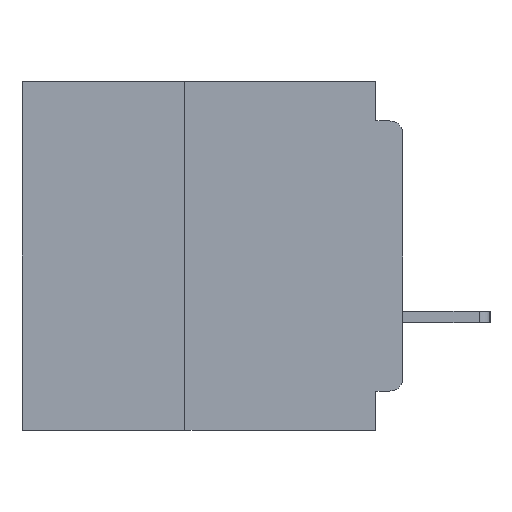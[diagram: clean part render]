
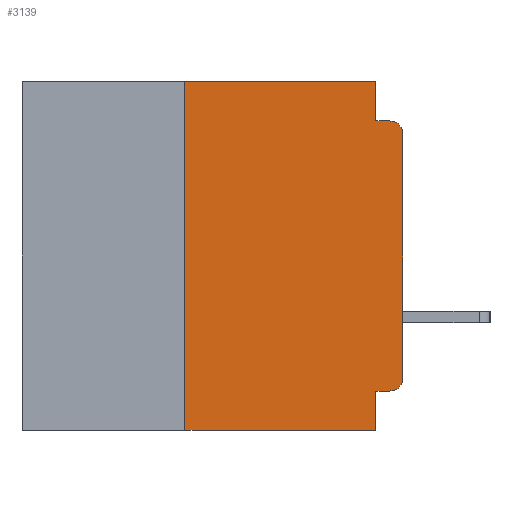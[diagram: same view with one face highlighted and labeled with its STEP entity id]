
A CAD part, left-side view. The second image highlights one B-rep face of the part: STEP entity #3139.
In plain terms, the highlighted planar face has unit normal (-1, 0, 0).
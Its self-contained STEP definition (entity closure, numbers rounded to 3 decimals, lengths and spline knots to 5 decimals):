
#1068 = DIRECTION ( 'NONE',  ( 0., 0., -1. ) ) ;
#1249 = CARTESIAN_POINT ( 'NONE',  ( 0., 0.031, -0.4 ) ) ;
#1463 = ORIENTED_EDGE ( 'NONE', *, *, #34857, .F. ) ;
#2091 = LINE ( 'NONE', #34393, #49224 ) ;
#2738 = VERTEX_POINT ( 'NONE', #10706 ) ;
#3139 = ADVANCED_FACE ( 'NONE', ( #7915 ), #60393, .F. ) ;
#3955 = VECTOR ( 'NONE', #50959, 39.37008 ) ;
#5659 = VECTOR ( 'NONE', #1068, 39.37008 ) ;
#5899 = VERTEX_POINT ( 'NONE', #46961 ) ;
#6038 = DIRECTION ( 'NONE',  ( 0., 0., -1. ) ) ;
#6344 = CARTESIAN_POINT ( 'NONE',  ( 0., 0.25, -0.4 ) ) ;
#7915 = FACE_OUTER_BOUND ( 'NONE', #13587, .T. ) ;
#7959 = CARTESIAN_POINT ( 'NONE',  ( 0., 0.015, -0.045 ) ) ;
#8168 = ORIENTED_EDGE ( 'NONE', *, *, #12337, .T. ) ;
#9077 = DIRECTION ( 'NONE',  ( 0., 0., 1. ) ) ;
#9308 = ORIENTED_EDGE ( 'NONE', *, *, #10342, .T. ) ;
#10342 = EDGE_CURVE ( 'NONE', #39145, #25069, #59137, .T. ) ;
#10361 = VERTEX_POINT ( 'NONE', #41801 ) ;
#10706 = CARTESIAN_POINT ( 'NONE',  ( 0., 0.031, 0. ) ) ;
#12289 = ORIENTED_EDGE ( 'NONE', *, *, #60987, .F. ) ;
#12337 = EDGE_CURVE ( 'NONE', #50974, #39145, #42805, .T. ) ;
#12587 = LINE ( 'NONE', #42976, #60980 ) ;
#13587 = EDGE_LOOP ( 'NONE', ( #8168, #9308, #1463, #35368, #51085, #40850, #23352, #12289, #43280, #24809 ) ) ;
#13833 = CARTESIAN_POINT ( 'NONE',  ( 0., 0., 0. ) ) ;
#14425 = EDGE_CURVE ( 'NONE', #45988, #5899, #2091, .T. ) ;
#14675 = DIRECTION ( 'NONE',  ( -1., 0., 0. ) ) ;
#15646 = DIRECTION ( 'NONE',  ( 0., -1., 0. ) ) ;
#16340 = VECTOR ( 'NONE', #9077, 39.37008 ) ;
#16522 = LINE ( 'NONE', #22852, #3955 ) ;
#17938 = CARTESIAN_POINT ( 'NONE',  ( 0., 0.015, -0.355 ) ) ;
#20840 = EDGE_CURVE ( 'NONE', #30914, #50974, #25900, .T. ) ;
#22852 = CARTESIAN_POINT ( 'NONE',  ( 0., 0.25, -0.4 ) ) ;
#22899 = CARTESIAN_POINT ( 'NONE',  ( 0., 0.015, -0.06 ) ) ;
#23352 = ORIENTED_EDGE ( 'NONE', *, *, #14425, .T. ) ;
#23419 = VECTOR ( 'NONE', #50188, 39.37008 ) ;
#24302 = DIRECTION ( 'NONE',  ( 0., 1., 0. ) ) ;
#24551 = AXIS2_PLACEMENT_3D ( 'NONE', #42814, #14675, #47511 ) ;
#24809 = ORIENTED_EDGE ( 'NONE', *, *, #20840, .T. ) ;
#25069 = VERTEX_POINT ( 'NONE', #7959 ) ;
#25653 = VERTEX_POINT ( 'NONE', #40621 ) ;
#25900 = CIRCLE ( 'NONE', #24551, 0.015 ) ;
#27038 = AXIS2_PLACEMENT_3D ( 'NONE', #46258, #45799, #39492 ) ;
#27456 = AXIS2_PLACEMENT_3D ( 'NONE', #22899, #55697, #27670 ) ;
#27570 = LINE ( 'NONE', #1249, #38583 ) ;
#27670 = DIRECTION ( 'NONE',  ( 0., 0., -1. ) ) ;
#28773 = EDGE_CURVE ( 'NONE', #25653, #2738, #45775, .T. ) ;
#30914 = VERTEX_POINT ( 'NONE', #17938 ) ;
#34393 = CARTESIAN_POINT ( 'NONE',  ( 0., 0.437, -0.4 ) ) ;
#34857 = EDGE_CURVE ( 'NONE', #60844, #25069, #60791, .T. ) ;
#35368 = ORIENTED_EDGE ( 'NONE', *, *, #35811, .F. ) ;
#35811 = EDGE_CURVE ( 'NONE', #2738, #60844, #54194, .T. ) ;
#36313 = VECTOR ( 'NONE', #58083, 39.37008 ) ;
#38583 = VECTOR ( 'NONE', #6038, 39.37008 ) ;
#38843 = CARTESIAN_POINT ( 'NONE',  ( 0., 0.031, 0. ) ) ;
#39145 = VERTEX_POINT ( 'NONE', #58120 ) ;
#39443 = EDGE_CURVE ( 'NONE', #45988, #25653, #16522, .T. ) ;
#39492 = DIRECTION ( 'NONE',  ( 0., 0., -1. ) ) ;
#40621 = CARTESIAN_POINT ( 'NONE',  ( 0., 0.25, 0. ) ) ;
#40850 = ORIENTED_EDGE ( 'NONE', *, *, #39443, .F. ) ;
#41415 = EDGE_CURVE ( 'NONE', #30914, #10361, #12587, .T. ) ;
#41801 = CARTESIAN_POINT ( 'NONE',  ( 0., 0.031, -0.355 ) ) ;
#42805 = LINE ( 'NONE', #13833, #16340 ) ;
#42814 = CARTESIAN_POINT ( 'NONE',  ( 0., 0.015, -0.34 ) ) ;
#42976 = CARTESIAN_POINT ( 'NONE',  ( 0., 0., -0.355 ) ) ;
#43280 = ORIENTED_EDGE ( 'NONE', *, *, #41415, .F. ) ;
#45775 = LINE ( 'NONE', #53403, #36313 ) ;
#45799 = DIRECTION ( 'NONE',  ( 1., 0., 0. ) ) ;
#45988 = VERTEX_POINT ( 'NONE', #6344 ) ;
#46258 = CARTESIAN_POINT ( 'NONE',  ( 0., 0.437, 0. ) ) ;
#46961 = CARTESIAN_POINT ( 'NONE',  ( 0., 0.031, -0.4 ) ) ;
#47511 = DIRECTION ( 'NONE',  ( 0., 0., -1. ) ) ;
#49224 = VECTOR ( 'NONE', #15646, 39.37008 ) ;
#50188 = DIRECTION ( 'NONE',  ( 0., -1., 0. ) ) ;
#50936 = CARTESIAN_POINT ( 'NONE',  ( 0., 0., -0.34 ) ) ;
#50959 = DIRECTION ( 'NONE',  ( 0., 0., 1. ) ) ;
#50974 = VERTEX_POINT ( 'NONE', #50936 ) ;
#51085 = ORIENTED_EDGE ( 'NONE', *, *, #28773, .F. ) ;
#53403 = CARTESIAN_POINT ( 'NONE',  ( 0., 0.437, 0. ) ) ;
#54194 = LINE ( 'NONE', #38843, #5659 ) ;
#55697 = DIRECTION ( 'NONE',  ( -1., 0., 0. ) ) ;
#56769 = CARTESIAN_POINT ( 'NONE',  ( 0., 0.031, -0.045 ) ) ;
#58083 = DIRECTION ( 'NONE',  ( 0., -1., 0. ) ) ;
#58120 = CARTESIAN_POINT ( 'NONE',  ( 0., 0., -0.06 ) ) ;
#59137 = CIRCLE ( 'NONE', #27456, 0.015 ) ;
#59566 = CARTESIAN_POINT ( 'NONE',  ( 0., 0., -0.045 ) ) ;
#60393 = PLANE ( 'NONE',  #27038 ) ;
#60791 = LINE ( 'NONE', #59566, #23419 ) ;
#60844 = VERTEX_POINT ( 'NONE', #56769 ) ;
#60980 = VECTOR ( 'NONE', #24302, 39.37008 ) ;
#60987 = EDGE_CURVE ( 'NONE', #10361, #5899, #27570, .T. ) ;
